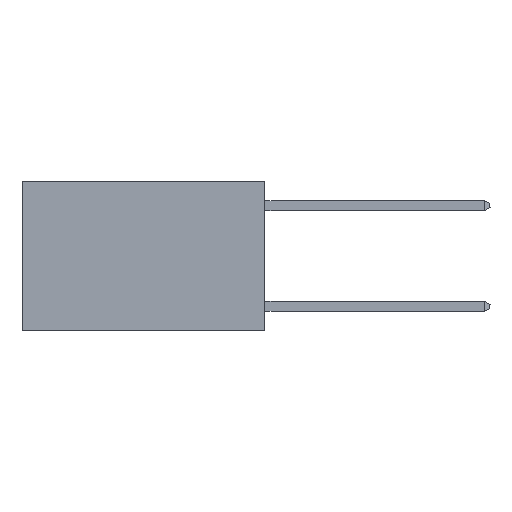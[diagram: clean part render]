
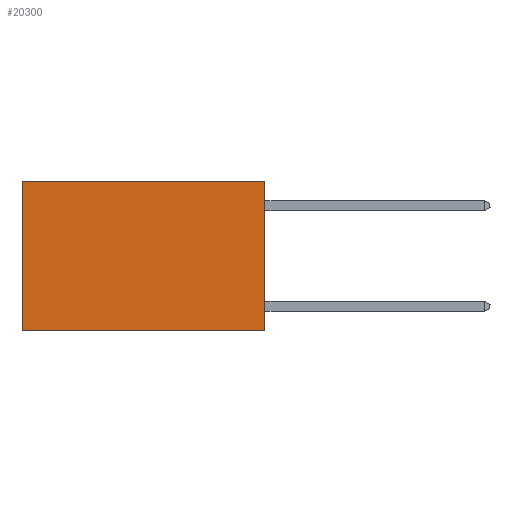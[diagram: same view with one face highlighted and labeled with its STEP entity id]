
A CAD part, left-side view. The second image highlights one B-rep face of the part: STEP entity #20300.
In plain terms, the highlighted planar face has unit normal (-1, 0, 0).
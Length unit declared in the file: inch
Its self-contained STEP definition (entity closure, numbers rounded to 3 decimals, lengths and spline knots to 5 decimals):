
#552 = EDGE_CURVE ( 'NONE', #4167, #7340, #16433, .T. ) ;
#818 = CARTESIAN_POINT ( 'NONE',  ( 0.2625, 0., 0. ) ) ;
#1100 = DIRECTION ( 'NONE',  ( 0., 1., 0. ) ) ;
#1307 = CARTESIAN_POINT ( 'NONE',  ( 0.2625, 0., -0.37 ) ) ;
#2486 = VECTOR ( 'NONE', #1100, 39.37008 ) ;
#2808 = EDGE_LOOP ( 'NONE', ( #19818, #15329, #18042, #11972 ) ) ;
#4167 = VERTEX_POINT ( 'NONE', #6727 ) ;
#4749 = DIRECTION ( 'NONE',  ( 0., 1., 0. ) ) ;
#5036 = CARTESIAN_POINT ( 'NONE',  ( 0.2625, 0.6, 0. ) ) ;
#5517 = CARTESIAN_POINT ( 'NONE',  ( 0.2625, 0., -0.37 ) ) ;
#6727 = CARTESIAN_POINT ( 'NONE',  ( 0.2625, 0., 0. ) ) ;
#6760 = LINE ( 'NONE', #15693, #8224 ) ;
#6761 = VERTEX_POINT ( 'NONE', #16384 ) ;
#7035 = CARTESIAN_POINT ( 'NONE',  ( 0.2625, 0., 0. ) ) ;
#7153 = LINE ( 'NONE', #1307, #2486 ) ;
#7340 = VERTEX_POINT ( 'NONE', #5517 ) ;
#8224 = VECTOR ( 'NONE', #4749, 39.37008 ) ;
#8625 = PLANE ( 'NONE',  #14423 ) ;
#8723 = CARTESIAN_POINT ( 'NONE',  ( 0.2625, 0.6, 0. ) ) ;
#10029 = VECTOR ( 'NONE', #13948, 39.37008 ) ;
#10439 = EDGE_CURVE ( 'NONE', #7340, #6761, #7153, .T. ) ;
#11235 = VECTOR ( 'NONE', #15093, 39.37008 ) ;
#11972 = ORIENTED_EDGE ( 'NONE', *, *, #13748, .T. ) ;
#12031 = DIRECTION ( 'NONE',  ( 0., 0., -1. ) ) ;
#12247 = FACE_OUTER_BOUND ( 'NONE', #2808, .T. ) ;
#13748 = EDGE_CURVE ( 'NONE', #4167, #18847, #6760, .T. ) ;
#13948 = DIRECTION ( 'NONE',  ( 0., 0., -1. ) ) ;
#14172 = EDGE_CURVE ( 'NONE', #18847, #6761, #14182, .T. ) ;
#14182 = LINE ( 'NONE', #8723, #11235 ) ;
#14423 = AXIS2_PLACEMENT_3D ( 'NONE', #818, #18080, #12031 ) ;
#15093 = DIRECTION ( 'NONE',  ( 0., 0., -1. ) ) ;
#15329 = ORIENTED_EDGE ( 'NONE', *, *, #10439, .F. ) ;
#15693 = CARTESIAN_POINT ( 'NONE',  ( 0.2625, 0., 0. ) ) ;
#16384 = CARTESIAN_POINT ( 'NONE',  ( 0.2625, 0.6, -0.37 ) ) ;
#16433 = LINE ( 'NONE', #7035, #10029 ) ;
#18042 = ORIENTED_EDGE ( 'NONE', *, *, #552, .F. ) ;
#18080 = DIRECTION ( 'NONE',  ( 1., 0., 0. ) ) ;
#18847 = VERTEX_POINT ( 'NONE', #5036 ) ;
#19818 = ORIENTED_EDGE ( 'NONE', *, *, #14172, .T. ) ;
#20300 = ADVANCED_FACE ( 'NONE', ( #12247 ), #8625, .F. ) ;
